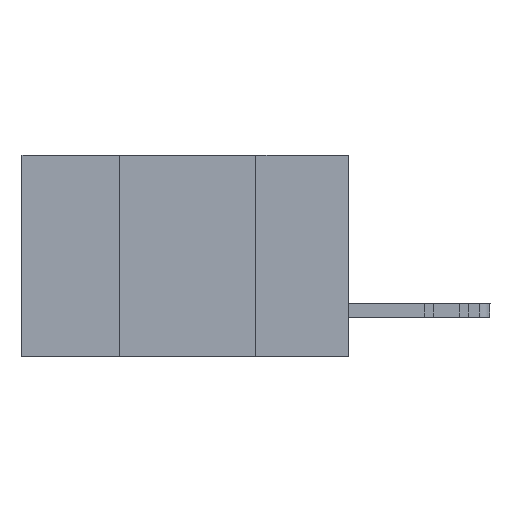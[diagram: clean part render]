
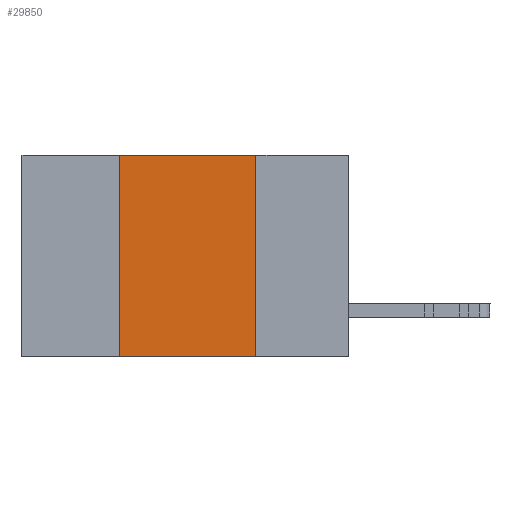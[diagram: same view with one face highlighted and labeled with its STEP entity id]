
A CAD part, left-side view. The second image highlights one B-rep face of the part: STEP entity #29850.
In plain terms, the highlighted planar face has unit normal (-1, 0, 0).
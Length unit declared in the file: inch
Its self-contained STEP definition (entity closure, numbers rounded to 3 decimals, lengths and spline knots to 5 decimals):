
#451 = DIRECTION ( 'NONE',  ( 0., 0., -1. ) ) ;
#481 = VECTOR ( 'NONE', #451, 39.37008 ) ;
#1501 = CARTESIAN_POINT ( 'NONE',  ( 0., 0.6, 0. ) ) ;
#4884 = LINE ( 'NONE', #32257, #24413 ) ;
#5164 = ORIENTED_EDGE ( 'NONE', *, *, #22412, .F. ) ;
#6188 = PLANE ( 'NONE',  #15177 ) ;
#7624 = LINE ( 'NONE', #22272, #32383 ) ;
#9821 = ORIENTED_EDGE ( 'NONE', *, *, #28462, .T. ) ;
#10618 = CARTESIAN_POINT ( 'NONE',  ( 0., 0.17, 0. ) ) ;
#11499 = DIRECTION ( 'NONE',  ( 0., -1., 0. ) ) ;
#11819 = DIRECTION ( 'NONE',  ( 0., -1., 0. ) ) ;
#13381 = DIRECTION ( 'NONE',  ( 0., 0., 1. ) ) ;
#13853 = ORIENTED_EDGE ( 'NONE', *, *, #22356, .F. ) ;
#13960 = DIRECTION ( 'NONE',  ( 1., 0., 0. ) ) ;
#15177 = AXIS2_PLACEMENT_3D ( 'NONE', #1501, #13960, #18893 ) ;
#17857 = VERTEX_POINT ( 'NONE', #22632 ) ;
#17865 = FACE_OUTER_BOUND ( 'NONE', #31068, .T. ) ;
#17910 = VERTEX_POINT ( 'NONE', #20603 ) ;
#18591 = VERTEX_POINT ( 'NONE', #31416 ) ;
#18893 = DIRECTION ( 'NONE',  ( 0., 0., -1. ) ) ;
#20465 = VERTEX_POINT ( 'NONE', #27011 ) ;
#20603 = CARTESIAN_POINT ( 'NONE',  ( 0., 0.17, -0.37 ) ) ;
#22272 = CARTESIAN_POINT ( 'NONE',  ( 0., 0.6, 0. ) ) ;
#22356 = EDGE_CURVE ( 'NONE', #18591, #17857, #29652, .T. ) ;
#22412 = EDGE_CURVE ( 'NONE', #20465, #17910, #22813, .T. ) ;
#22632 = CARTESIAN_POINT ( 'NONE',  ( 0., 0.42, 0. ) ) ;
#22813 = LINE ( 'NONE', #10618, #481 ) ;
#24413 = VECTOR ( 'NONE', #11499, 39.37008 ) ;
#26049 = VECTOR ( 'NONE', #13381, 39.37008 ) ;
#26133 = CARTESIAN_POINT ( 'NONE',  ( 0., 0.42, 0. ) ) ;
#27011 = CARTESIAN_POINT ( 'NONE',  ( 0., 0.17, 0. ) ) ;
#28462 = EDGE_CURVE ( 'NONE', #18591, #17910, #4884, .T. ) ;
#29006 = ORIENTED_EDGE ( 'NONE', *, *, #33081, .F. ) ;
#29652 = LINE ( 'NONE', #26133, #26049 ) ;
#29850 = ADVANCED_FACE ( 'NONE', ( #17865 ), #6188, .F. ) ;
#31068 = EDGE_LOOP ( 'NONE', ( #5164, #29006, #13853, #9821 ) ) ;
#31416 = CARTESIAN_POINT ( 'NONE',  ( 0., 0.42, -0.37 ) ) ;
#32257 = CARTESIAN_POINT ( 'NONE',  ( 0., 0.6, -0.37 ) ) ;
#32383 = VECTOR ( 'NONE', #11819, 39.37008 ) ;
#33081 = EDGE_CURVE ( 'NONE', #17857, #20465, #7624, .T. ) ;
